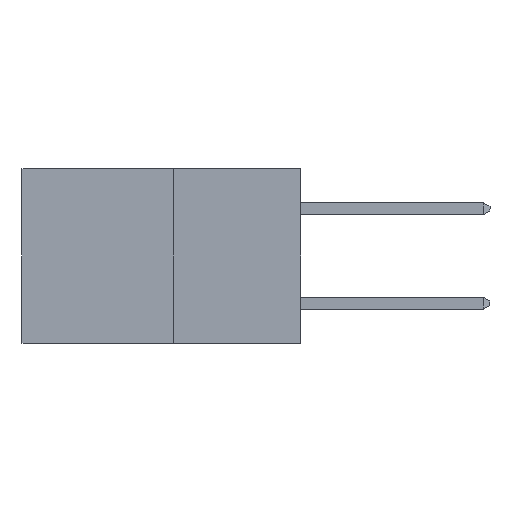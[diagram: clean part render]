
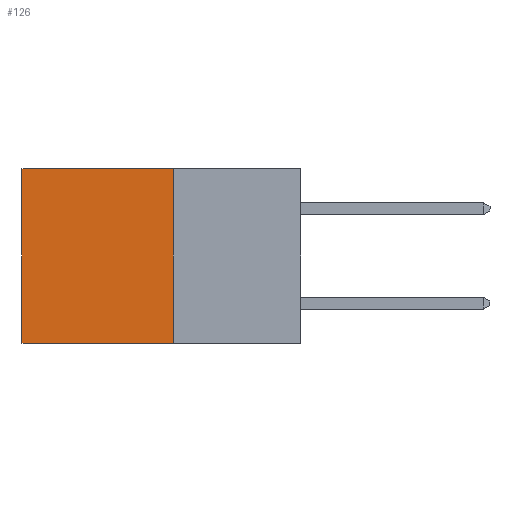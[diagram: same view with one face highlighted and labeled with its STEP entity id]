
A CAD part, left-side view. The second image highlights one B-rep face of the part: STEP entity #126.
In plain terms, the highlighted planar face has unit normal (-1, 0, 0).
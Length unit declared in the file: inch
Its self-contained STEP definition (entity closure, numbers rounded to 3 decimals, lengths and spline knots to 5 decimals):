
#126 = ADVANCED_FACE ( 'NONE', ( #6373 ), #2953, .F. ) ;
#411 = ORIENTED_EDGE ( 'NONE', *, *, #2722, .F. ) ;
#827 = LINE ( 'NONE', #1942, #2673 ) ;
#900 = DIRECTION ( 'NONE',  ( 1., 0., 0. ) ) ;
#1005 = LINE ( 'NONE', #7569, #7554 ) ;
#1188 = EDGE_CURVE ( 'NONE', #2049, #6258, #2952, .T. ) ;
#1223 = EDGE_CURVE ( 'NONE', #2049, #7633, #827, .T. ) ;
#1312 = DIRECTION ( 'NONE',  ( 0., 1., 0. ) ) ;
#1942 = CARTESIAN_POINT ( 'NONE',  ( 0.277, 0.27, -0.37 ) ) ;
#1967 = DIRECTION ( 'NONE',  ( 0., 0., -1. ) ) ;
#2049 = VERTEX_POINT ( 'NONE', #6026 ) ;
#2407 = ORIENTED_EDGE ( 'NONE', *, *, #8102, .T. ) ;
#2673 = VECTOR ( 'NONE', #1967, 39.37008 ) ;
#2722 = EDGE_CURVE ( 'NONE', #7633, #5262, #1005, .T. ) ;
#2944 = VECTOR ( 'NONE', #4014, 39.37008 ) ;
#2952 = LINE ( 'NONE', #4733, #3148 ) ;
#2953 = PLANE ( 'NONE',  #3242 ) ;
#3148 = VECTOR ( 'NONE', #1312, 39.37008 ) ;
#3170 = ORIENTED_EDGE ( 'NONE', *, *, #1188, .T. ) ;
#3242 = AXIS2_PLACEMENT_3D ( 'NONE', #7981, #900, #8097 ) ;
#3982 = CARTESIAN_POINT ( 'NONE',  ( 0.277, 0.59, -0.37 ) ) ;
#4014 = DIRECTION ( 'NONE',  ( 0., 0., -1. ) ) ;
#4350 = ORIENTED_EDGE ( 'NONE', *, *, #1223, .F. ) ;
#4733 = CARTESIAN_POINT ( 'NONE',  ( 0.277, 0.27, 0. ) ) ;
#5262 = VERTEX_POINT ( 'NONE', #7852 ) ;
#5499 = CARTESIAN_POINT ( 'NONE',  ( 0.277, 0.59, 0. ) ) ;
#5654 = CARTESIAN_POINT ( 'NONE',  ( 0.277, 0.27, -0.37 ) ) ;
#5984 = EDGE_LOOP ( 'NONE', ( #2407, #411, #4350, #3170 ) ) ;
#6026 = CARTESIAN_POINT ( 'NONE',  ( 0.277, 0.27, 0. ) ) ;
#6258 = VERTEX_POINT ( 'NONE', #5499 ) ;
#6373 = FACE_OUTER_BOUND ( 'NONE', #5984, .T. ) ;
#6588 = DIRECTION ( 'NONE',  ( 0., 1., 0. ) ) ;
#7554 = VECTOR ( 'NONE', #6588, 39.37008 ) ;
#7569 = CARTESIAN_POINT ( 'NONE',  ( 0.277, 0.27, -0.37 ) ) ;
#7633 = VERTEX_POINT ( 'NONE', #5654 ) ;
#7852 = CARTESIAN_POINT ( 'NONE',  ( 0.277, 0.59, -0.37 ) ) ;
#7981 = CARTESIAN_POINT ( 'NONE',  ( 0.277, 0.27, -0.37 ) ) ;
#8018 = LINE ( 'NONE', #3982, #2944 ) ;
#8097 = DIRECTION ( 'NONE',  ( 0., 0., -1. ) ) ;
#8102 = EDGE_CURVE ( 'NONE', #6258, #5262, #8018, .T. ) ;
